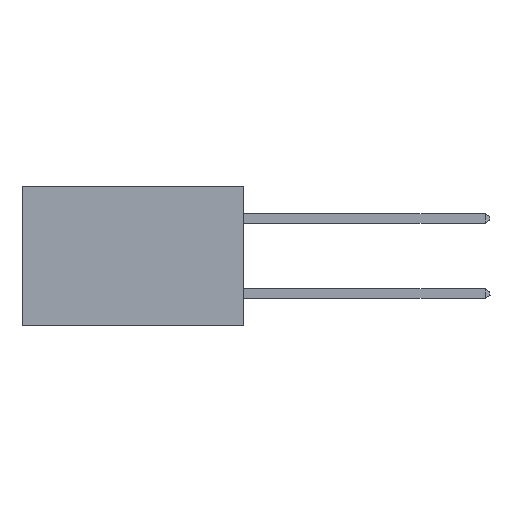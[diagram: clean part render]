
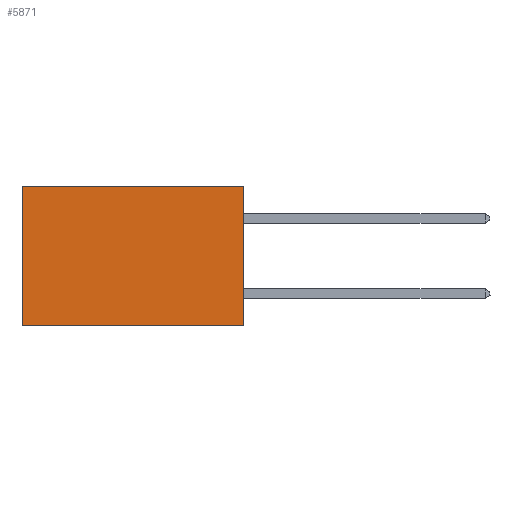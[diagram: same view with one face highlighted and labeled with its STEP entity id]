
A CAD part, left-side view. The second image highlights one B-rep face of the part: STEP entity #5871.
In plain terms, the highlighted planar face has unit normal (-1, 0, 0).
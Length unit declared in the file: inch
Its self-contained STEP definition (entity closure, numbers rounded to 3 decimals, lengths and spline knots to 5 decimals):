
#1092 = CARTESIAN_POINT ( 'NONE',  ( 0.277, 0., 0. ) ) ;
#1585 = ORIENTED_EDGE ( 'NONE', *, *, #22708, .F. ) ;
#2301 = CARTESIAN_POINT ( 'NONE',  ( 0.277, 0., -0.37 ) ) ;
#2505 = AXIS2_PLACEMENT_3D ( 'NONE', #8871, #8775, #8715 ) ;
#3049 = VERTEX_POINT ( 'NONE', #5668 ) ;
#4434 = CARTESIAN_POINT ( 'NONE',  ( 0.277, 0., 0. ) ) ;
#5317 = ORIENTED_EDGE ( 'NONE', *, *, #10948, .T. ) ;
#5460 = CARTESIAN_POINT ( 'NONE',  ( 0.277, 0., -0.37 ) ) ;
#5668 = CARTESIAN_POINT ( 'NONE',  ( 0.277, 0.59, 0. ) ) ;
#5871 = ADVANCED_FACE ( 'NONE', ( #16592 ), #8798, .F. ) ;
#6456 = DIRECTION ( 'NONE',  ( 0., 1., 0. ) ) ;
#7455 = VERTEX_POINT ( 'NONE', #18799 ) ;
#7871 = ORIENTED_EDGE ( 'NONE', *, *, #15309, .F. ) ;
#8317 = LINE ( 'NONE', #2301, #12645 ) ;
#8715 = DIRECTION ( 'NONE',  ( 0., 0., -1. ) ) ;
#8775 = DIRECTION ( 'NONE',  ( 1., 0., 0. ) ) ;
#8798 = PLANE ( 'NONE',  #2505 ) ;
#8871 = CARTESIAN_POINT ( 'NONE',  ( 0.277, 0., -0.37 ) ) ;
#9052 = VERTEX_POINT ( 'NONE', #1092 ) ;
#9069 = LINE ( 'NONE', #14371, #23187 ) ;
#9883 = DIRECTION ( 'NONE',  ( 0., 1., 0. ) ) ;
#10738 = DIRECTION ( 'NONE',  ( 0., 0., -1. ) ) ;
#10948 = EDGE_CURVE ( 'NONE', #3049, #7455, #16082, .T. ) ;
#12645 = VECTOR ( 'NONE', #9883, 39.37008 ) ;
#13086 = EDGE_CURVE ( 'NONE', #9052, #3049, #14093, .T. ) ;
#13182 = EDGE_LOOP ( 'NONE', ( #5317, #1585, #7871, #20860 ) ) ;
#14093 = LINE ( 'NONE', #4434, #23295 ) ;
#14371 = CARTESIAN_POINT ( 'NONE',  ( 0.277, 0., -0.37 ) ) ;
#15309 = EDGE_CURVE ( 'NONE', #9052, #15439, #9069, .T. ) ;
#15439 = VERTEX_POINT ( 'NONE', #5460 ) ;
#16082 = LINE ( 'NONE', #19922, #20401 ) ;
#16592 = FACE_OUTER_BOUND ( 'NONE', #13182, .T. ) ;
#18072 = DIRECTION ( 'NONE',  ( 0., 0., -1. ) ) ;
#18799 = CARTESIAN_POINT ( 'NONE',  ( 0.277, 0.59, -0.37 ) ) ;
#19922 = CARTESIAN_POINT ( 'NONE',  ( 0.277, 0.59, -0.37 ) ) ;
#20401 = VECTOR ( 'NONE', #10738, 39.37008 ) ;
#20860 = ORIENTED_EDGE ( 'NONE', *, *, #13086, .T. ) ;
#22708 = EDGE_CURVE ( 'NONE', #15439, #7455, #8317, .T. ) ;
#23187 = VECTOR ( 'NONE', #18072, 39.37008 ) ;
#23295 = VECTOR ( 'NONE', #6456, 39.37008 ) ;
